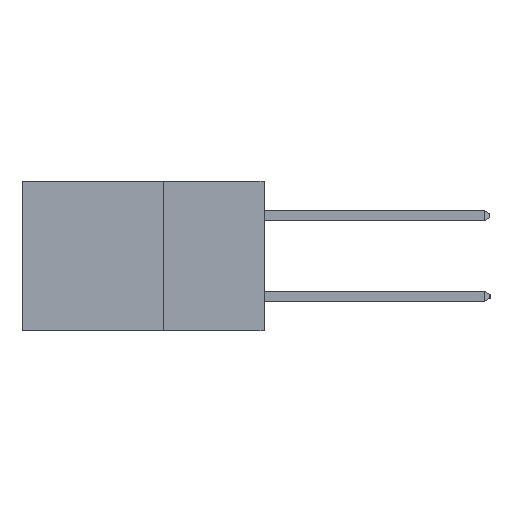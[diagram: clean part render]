
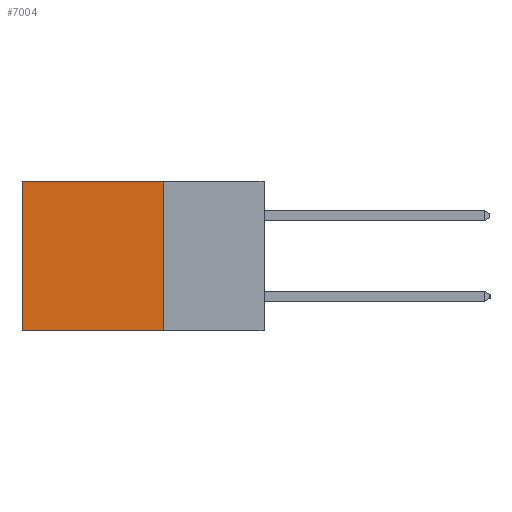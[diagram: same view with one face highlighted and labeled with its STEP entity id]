
A CAD part, left-side view. The second image highlights one B-rep face of the part: STEP entity #7004.
In plain terms, the highlighted planar face has unit normal (-1, 0, 0).
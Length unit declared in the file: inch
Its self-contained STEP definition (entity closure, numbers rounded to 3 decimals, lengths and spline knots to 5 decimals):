
#319 = VERTEX_POINT ( 'NONE', #13143 ) ;
#1237 = CARTESIAN_POINT ( 'NONE',  ( 0.2615, 0.6, -0.37 ) ) ;
#1674 = VECTOR ( 'NONE', #14474, 39.37008 ) ;
#2211 = VECTOR ( 'NONE', #6050, 39.37008 ) ;
#2452 = ORIENTED_EDGE ( 'NONE', *, *, #13194, .T. ) ;
#2636 = VERTEX_POINT ( 'NONE', #14664 ) ;
#2684 = LINE ( 'NONE', #5265, #12381 ) ;
#2799 = CARTESIAN_POINT ( 'NONE',  ( 0.2615, 0.25, -0.37 ) ) ;
#3388 = VECTOR ( 'NONE', #12344, 39.37008 ) ;
#4771 = CARTESIAN_POINT ( 'NONE',  ( 0.2615, 0.6, -0.37 ) ) ;
#5175 = LINE ( 'NONE', #4771, #2211 ) ;
#5265 = CARTESIAN_POINT ( 'NONE',  ( 0.2615, 0.25, 0. ) ) ;
#5333 = PLANE ( 'NONE',  #12888 ) ;
#6050 = DIRECTION ( 'NONE',  ( 0., 0., -1. ) ) ;
#6613 = DIRECTION ( 'NONE',  ( 0., 0., -1. ) ) ;
#6881 = ORIENTED_EDGE ( 'NONE', *, *, #10332, .T. ) ;
#7004 = ADVANCED_FACE ( 'NONE', ( #12398 ), #5333, .F. ) ;
#7391 = EDGE_CURVE ( 'NONE', #2636, #13008, #13510, .T. ) ;
#8597 = VERTEX_POINT ( 'NONE', #1237 ) ;
#9778 = EDGE_LOOP ( 'NONE', ( #2452, #12136, #13992, #6881 ) ) ;
#10332 = EDGE_CURVE ( 'NONE', #2636, #319, #2684, .T. ) ;
#11062 = CARTESIAN_POINT ( 'NONE',  ( 0.2615, 0.25, -0.37 ) ) ;
#11551 = EDGE_CURVE ( 'NONE', #13008, #8597, #11744, .T. ) ;
#11744 = LINE ( 'NONE', #13184, #1674 ) ;
#12136 = ORIENTED_EDGE ( 'NONE', *, *, #11551, .F. ) ;
#12344 = DIRECTION ( 'NONE',  ( 0., 0., -1. ) ) ;
#12381 = VECTOR ( 'NONE', #12866, 39.37008 ) ;
#12398 = FACE_OUTER_BOUND ( 'NONE', #9778, .T. ) ;
#12866 = DIRECTION ( 'NONE',  ( 0., 1., 0. ) ) ;
#12888 = AXIS2_PLACEMENT_3D ( 'NONE', #2799, #14219, #6613 ) ;
#13008 = VERTEX_POINT ( 'NONE', #14587 ) ;
#13143 = CARTESIAN_POINT ( 'NONE',  ( 0.2615, 0.6, 0. ) ) ;
#13184 = CARTESIAN_POINT ( 'NONE',  ( 0.2615, 0.25, -0.37 ) ) ;
#13194 = EDGE_CURVE ( 'NONE', #319, #8597, #5175, .T. ) ;
#13510 = LINE ( 'NONE', #11062, #3388 ) ;
#13992 = ORIENTED_EDGE ( 'NONE', *, *, #7391, .F. ) ;
#14219 = DIRECTION ( 'NONE',  ( 1., 0., 0. ) ) ;
#14474 = DIRECTION ( 'NONE',  ( 0., 1., 0. ) ) ;
#14587 = CARTESIAN_POINT ( 'NONE',  ( 0.2615, 0.25, -0.37 ) ) ;
#14664 = CARTESIAN_POINT ( 'NONE',  ( 0.2615, 0.25, 0. ) ) ;
